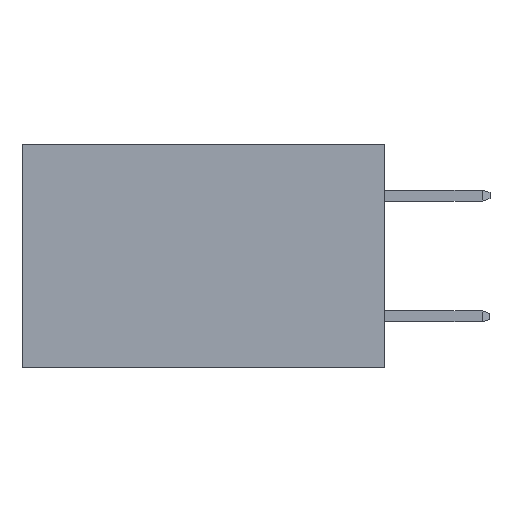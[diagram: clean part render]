
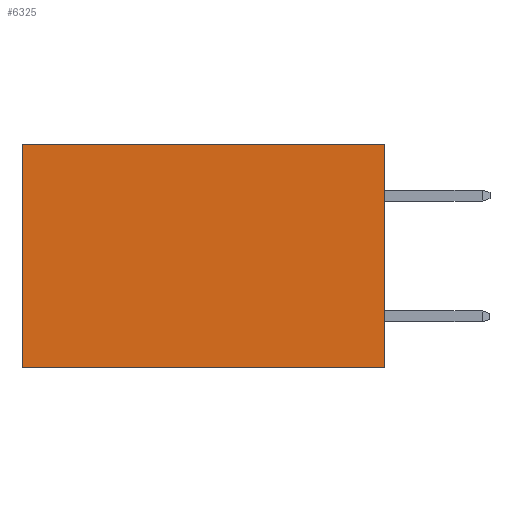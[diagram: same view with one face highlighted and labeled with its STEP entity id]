
A CAD part, left-side view. The second image highlights one B-rep face of the part: STEP entity #6325.
In plain terms, the highlighted planar face has unit normal (-1, 0, 0).
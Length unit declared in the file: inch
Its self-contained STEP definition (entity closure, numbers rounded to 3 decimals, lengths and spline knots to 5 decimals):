
#644 = EDGE_LOOP ( 'NONE', ( #1169, #5042, #4812, #4307 ) ) ;
#653 = LINE ( 'NONE', #1358, #2826 ) ;
#787 = LINE ( 'NONE', #4883, #4417 ) ;
#939 = CARTESIAN_POINT ( 'NONE',  ( 0.2615, 0.6, 0. ) ) ;
#982 = CARTESIAN_POINT ( 'NONE',  ( 0.2615, 0., -0.37 ) ) ;
#1169 = ORIENTED_EDGE ( 'NONE', *, *, #7500, .T. ) ;
#1182 = VECTOR ( 'NONE', #3226, 39.37008 ) ;
#1283 = CARTESIAN_POINT ( 'NONE',  ( 0.2615, 0., 0. ) ) ;
#1358 = CARTESIAN_POINT ( 'NONE',  ( 0.2615, 0., -0.37 ) ) ;
#1520 = DIRECTION ( 'NONE',  ( 0., 0., -1. ) ) ;
#2486 = LINE ( 'NONE', #8660, #1182 ) ;
#2786 = EDGE_CURVE ( 'NONE', #5476, #5014, #7423, .T. ) ;
#2802 = EDGE_CURVE ( 'NONE', #5476, #7516, #653, .T. ) ;
#2826 = VECTOR ( 'NONE', #5583, 39.37008 ) ;
#3226 = DIRECTION ( 'NONE',  ( 0., 0., -1. ) ) ;
#3989 = VECTOR ( 'NONE', #7504, 39.37008 ) ;
#4040 = VERTEX_POINT ( 'NONE', #5297 ) ;
#4307 = ORIENTED_EDGE ( 'NONE', *, *, #2786, .T. ) ;
#4417 = VECTOR ( 'NONE', #7174, 39.37008 ) ;
#4812 = ORIENTED_EDGE ( 'NONE', *, *, #2802, .F. ) ;
#4883 = CARTESIAN_POINT ( 'NONE',  ( 0.2615, 0., -0.37 ) ) ;
#5014 = VERTEX_POINT ( 'NONE', #939 ) ;
#5042 = ORIENTED_EDGE ( 'NONE', *, *, #5933, .F. ) ;
#5297 = CARTESIAN_POINT ( 'NONE',  ( 0.2615, 0.6, -0.37 ) ) ;
#5476 = VERTEX_POINT ( 'NONE', #8445 ) ;
#5583 = DIRECTION ( 'NONE',  ( 0., 0., -1. ) ) ;
#5933 = EDGE_CURVE ( 'NONE', #7516, #4040, #787, .T. ) ;
#6325 = ADVANCED_FACE ( 'NONE', ( #6986 ), #7793, .F. ) ;
#6823 = CARTESIAN_POINT ( 'NONE',  ( 0.2615, 0., -0.37 ) ) ;
#6986 = FACE_OUTER_BOUND ( 'NONE', #644, .T. ) ;
#7118 = AXIS2_PLACEMENT_3D ( 'NONE', #982, #7665, #1520 ) ;
#7174 = DIRECTION ( 'NONE',  ( 0., 1., 0. ) ) ;
#7423 = LINE ( 'NONE', #1283, #3989 ) ;
#7500 = EDGE_CURVE ( 'NONE', #5014, #4040, #2486, .T. ) ;
#7504 = DIRECTION ( 'NONE',  ( 0., 1., 0. ) ) ;
#7516 = VERTEX_POINT ( 'NONE', #6823 ) ;
#7665 = DIRECTION ( 'NONE',  ( 1., 0., 0. ) ) ;
#7793 = PLANE ( 'NONE',  #7118 ) ;
#8445 = CARTESIAN_POINT ( 'NONE',  ( 0.2615, 0., 0. ) ) ;
#8660 = CARTESIAN_POINT ( 'NONE',  ( 0.2615, 0.6, -0.37 ) ) ;
